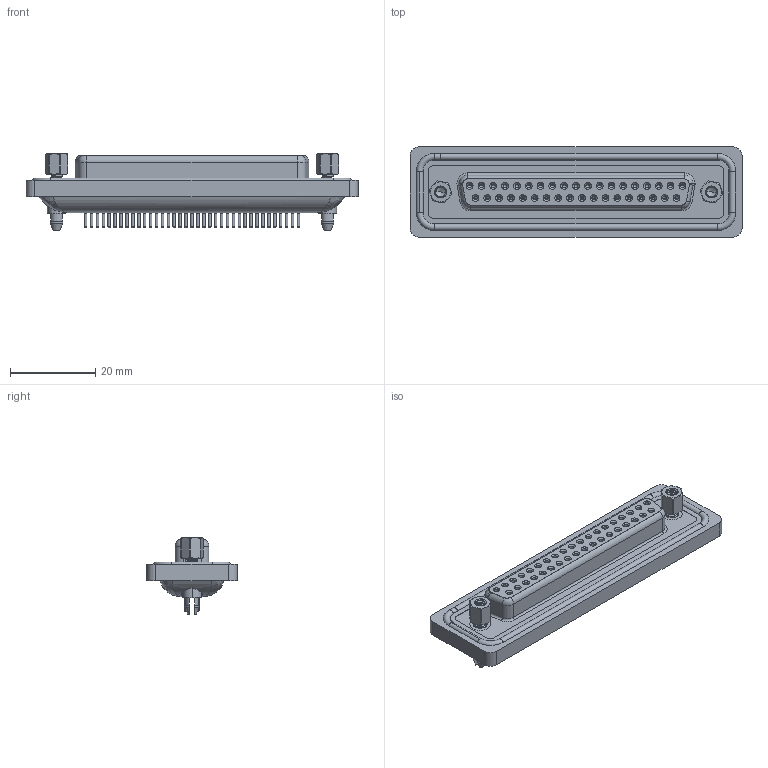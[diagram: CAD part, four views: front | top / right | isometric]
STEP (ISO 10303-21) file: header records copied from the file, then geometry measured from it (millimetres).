
FILE_DESCRIPTION (( 'STEP AP203' ), '1' );
FILE_NAME ('628-W37-620-013.STEP', '2024-03-21T19:42:16', ( '' ), ( '' ), 'SwSTEP 2.0', 'SolidWorks 2023', '' );
FILE_SCHEMA (( 'CONFIG_CONTROL_DESIGN' ));
Length unit declared in the file: millimetre
Products named in the file (8): 628W Housing_37 Contacts; 628W 4-40 Hex Standoff; 628-W37-620-013; 628W Shell Front_37 Contacts; 628W Contact Row 1_20; 628W Waterproof Housing_37 Contacts BL; 628W 4-40 Threaded Boardlock; 628W Contact Row 2_20
Assembly tree (44 placements, depth 2):
  628-W37-620-013
    628W Housing_37 Contacts
    628W Shell Front_37 Contacts
    628W Contact Row 1_20  x19
    628W Contact Row 2_20  x18
    628W 4-40 Threaded Boardlock  x2
    628W Waterproof Housing_37 Contacts BL
    628W 4-40 Hex Standoff  x2
Bounding box: 77.8 x 21.1 x 17.95 mm (x, y, z)
Volume: 11032.9 mm3; surface area: 18127.3 mm2
Topology: 45 solids, 45 shells, 2580 faces, 6090 edges, 3761 vertices
Faces by surface type: cylinder 1029, plane 670, torus 568, cone 291, bspline 22
Entity records: 35172 total; most frequent: CARTESIAN_POINT 9534, DIRECTION 5406, ORIENTED_EDGE 4654, EDGE_CURVE 2327, AXIS2_PLACEMENT_3D 2273, VERTEX_POINT 1489, EDGE_LOOP 1282, CIRCLE 1251
